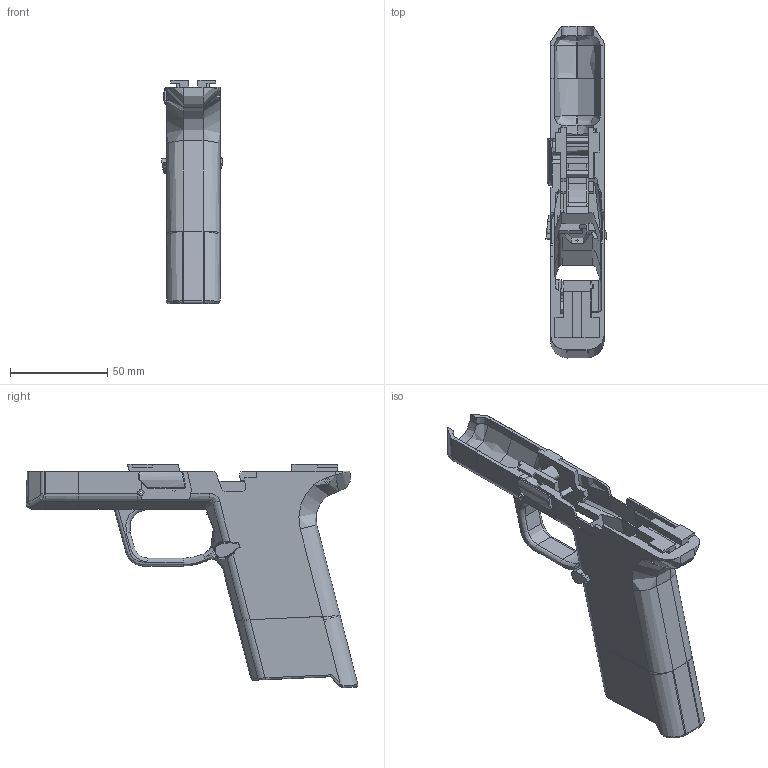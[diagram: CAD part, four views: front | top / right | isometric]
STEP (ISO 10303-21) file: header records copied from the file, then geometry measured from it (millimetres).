
FILE_DESCRIPTION(/* description */ (''),/* implementation_level */ '2;1');
FILE_NAME(/* name */ 'M&P 9 Assembly.step',/* time_stamp */ '2021-11-03T09:16:13-04:00',/* author */ (''),/* organization */ (''),/* preprocessor_version */ 'ST-DEVELOPER v18.1',/* originating_system */ 'Autodesk Translation Framework v10.10.0.1391',/* authorisation */ '');
FILE_SCHEMA (('AUTOMOTIVE_DESIGN { 1 0 10303 214 3 1 1 }'));
Length unit declared in the file: millimetre
Products named in the file (13): M&P 9 Reference; Rear Fire Control Group Pin; Front Locking Block Group Pin; Trigger Pin; Locking Block; Disassembly Lug; Rear Fire Control Group; Frame; Trigger Guard and Magwell; Fitment Section; Nose; Magazine Release Button; Full-Size Magwell Body
Assembly tree (12 placements, depth 4):
  M&P 9 Reference
    Rear Fire Control Group Pin
    Front Locking Block Group Pin
    Trigger Pin
    Locking Block
    Disassembly Lug
    Rear Fire Control Group
    Frame
      Trigger Guard and Magwell
      Fitment Section
        Nose
      Magazine Release Button
      Full-Size Magwell Body
Bounding box: 30.85 x 170.13 x 114.63 mm (x, y, z)
Volume: 102642.2 mm3; surface area: 57535.8 mm2
Topology: 12 solids, 12 shells, 630 faces, 1721 edges, 1102 vertices
Faces by surface type: plane 334, cylinder 194, bspline 80, torus 17, sphere 4, cone 1
Full cylindrical faces by diameter (mm): 1.35 x2, 1.5 x3, 3.15 x2, 3.18 x3, 3.2 x2, 3.361 x2, 3.5 x1, 3.55 x4, 4.7 x2, 6.3 x1, 7.7 x1, 8.8 x1, 9 x2
Entity records: 22907 total; most frequent: CARTESIAN_POINT 6643, ORIENTED_EDGE 3434, DIRECTION 3209, EDGE_CURVE 1717, VERTEX_POINT 1102, LINE 1077, VECTOR 1077, AXIS2_PLACEMENT_3D 1066
